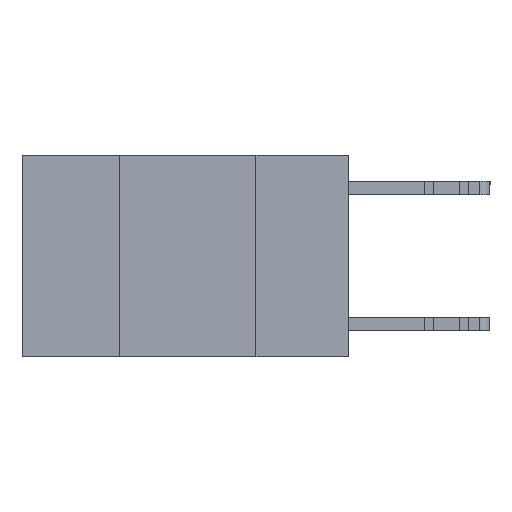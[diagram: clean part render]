
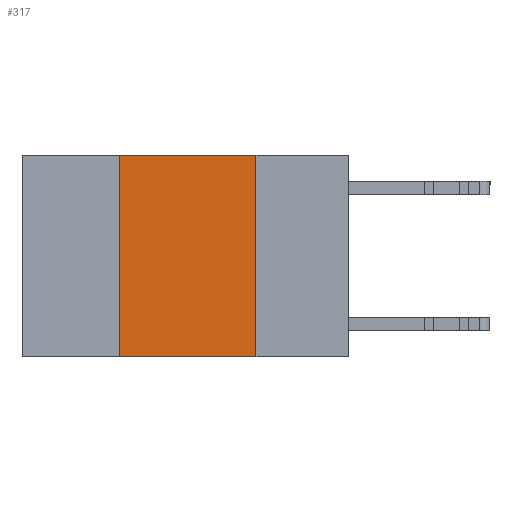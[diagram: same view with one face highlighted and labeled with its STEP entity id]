
A CAD part, left-side view. The second image highlights one B-rep face of the part: STEP entity #317.
In plain terms, the highlighted planar face has unit normal (-1, 0, 0).
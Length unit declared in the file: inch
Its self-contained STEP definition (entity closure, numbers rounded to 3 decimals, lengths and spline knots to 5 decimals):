
#317 = ADVANCED_FACE ( 'NONE', ( #28363 ), #11042, .F. ) ;
#936 = CARTESIAN_POINT ( 'NONE',  ( 0., 0.17, 0. ) ) ;
#1421 = VECTOR ( 'NONE', #9098, 39.37008 ) ;
#3732 = VECTOR ( 'NONE', #25328, 39.37008 ) ;
#3844 = DIRECTION ( 'NONE',  ( 1., 0., 0. ) ) ;
#6547 = LINE ( 'NONE', #28672, #1421 ) ;
#8041 = VERTEX_POINT ( 'NONE', #936 ) ;
#8369 = CARTESIAN_POINT ( 'NONE',  ( 0., 0.17, -0.37 ) ) ;
#8537 = VERTEX_POINT ( 'NONE', #8369 ) ;
#9098 = DIRECTION ( 'NONE',  ( 0., 0., 1. ) ) ;
#9110 = CARTESIAN_POINT ( 'NONE',  ( 0., 0.6, 0. ) ) ;
#9376 = VECTOR ( 'NONE', #18738, 39.37008 ) ;
#9696 = ORIENTED_EDGE ( 'NONE', *, *, #24800, .F. ) ;
#11042 = PLANE ( 'NONE',  #13437 ) ;
#12006 = CARTESIAN_POINT ( 'NONE',  ( 0., 0.6, -0.37 ) ) ;
#12514 = ORIENTED_EDGE ( 'NONE', *, *, #21097, .F. ) ;
#12914 = VERTEX_POINT ( 'NONE', #23976 ) ;
#13250 = ORIENTED_EDGE ( 'NONE', *, *, #14967, .T. ) ;
#13437 = AXIS2_PLACEMENT_3D ( 'NONE', #9110, #3844, #20809 ) ;
#13596 = EDGE_CURVE ( 'NONE', #8041, #8537, #23064, .T. ) ;
#14967 = EDGE_CURVE ( 'NONE', #12914, #8537, #21778, .T. ) ;
#15000 = CARTESIAN_POINT ( 'NONE',  ( 0., 0.6, 0. ) ) ;
#15846 = EDGE_LOOP ( 'NONE', ( #17063, #9696, #12514, #13250 ) ) ;
#17063 = ORIENTED_EDGE ( 'NONE', *, *, #13596, .F. ) ;
#18738 = DIRECTION ( 'NONE',  ( 0., -1., 0. ) ) ;
#20809 = DIRECTION ( 'NONE',  ( 0., 0., -1. ) ) ;
#21097 = EDGE_CURVE ( 'NONE', #12914, #30713, #6547, .T. ) ;
#21778 = LINE ( 'NONE', #12006, #9376 ) ;
#22200 = DIRECTION ( 'NONE',  ( 0., -1., 0. ) ) ;
#22502 = LINE ( 'NONE', #15000, #27609 ) ;
#23064 = LINE ( 'NONE', #25493, #3732 ) ;
#23976 = CARTESIAN_POINT ( 'NONE',  ( 0., 0.42, -0.37 ) ) ;
#24800 = EDGE_CURVE ( 'NONE', #30713, #8041, #22502, .T. ) ;
#25328 = DIRECTION ( 'NONE',  ( 0., 0., -1. ) ) ;
#25493 = CARTESIAN_POINT ( 'NONE',  ( 0., 0.17, 0. ) ) ;
#27609 = VECTOR ( 'NONE', #22200, 39.37008 ) ;
#27642 = CARTESIAN_POINT ( 'NONE',  ( 0., 0.42, 0. ) ) ;
#28363 = FACE_OUTER_BOUND ( 'NONE', #15846, .T. ) ;
#28672 = CARTESIAN_POINT ( 'NONE',  ( 0., 0.42, 0. ) ) ;
#30713 = VERTEX_POINT ( 'NONE', #27642 ) ;
